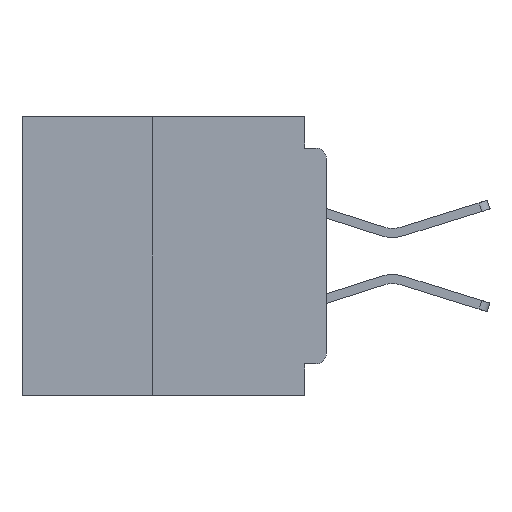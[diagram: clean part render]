
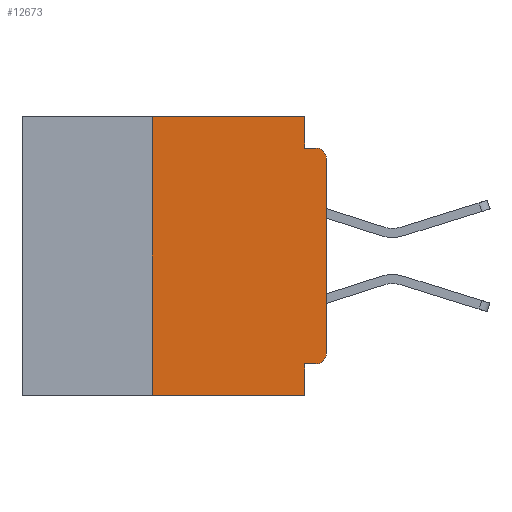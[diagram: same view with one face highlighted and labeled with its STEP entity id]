
A CAD part, left-side view. The second image highlights one B-rep face of the part: STEP entity #12673.
In plain terms, the highlighted planar face has unit normal (-1, 0, 0).
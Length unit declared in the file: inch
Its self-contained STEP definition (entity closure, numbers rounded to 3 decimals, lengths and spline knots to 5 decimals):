
#112 = CARTESIAN_POINT ( 'NONE',  ( 0., 0., -0.355 ) ) ;
#574 = CARTESIAN_POINT ( 'NONE',  ( 0., 0.437, -0.4 ) ) ;
#631 = VERTEX_POINT ( 'NONE', #1686 ) ;
#1043 = EDGE_CURVE ( 'NONE', #2421, #39814, #21181, .T. ) ;
#1280 = VECTOR ( 'NONE', #12761, 39.37008 ) ;
#1314 = CARTESIAN_POINT ( 'NONE',  ( 0., 0.015, -0.045 ) ) ;
#1686 = CARTESIAN_POINT ( 'NONE',  ( 0., 0.031, -0.355 ) ) ;
#2421 = VERTEX_POINT ( 'NONE', #5644 ) ;
#2426 = LINE ( 'NONE', #34821, #18251 ) ;
#3093 = CARTESIAN_POINT ( 'NONE',  ( 0., 0.25, -0.4 ) ) ;
#3097 = CARTESIAN_POINT ( 'NONE',  ( 0., 0.031, -0.4 ) ) ;
#3476 = CARTESIAN_POINT ( 'NONE',  ( 0., 0.015, -0.06 ) ) ;
#3678 = EDGE_CURVE ( 'NONE', #27109, #631, #16593, .T. ) ;
#3680 = CARTESIAN_POINT ( 'NONE',  ( 0., 0.031, 0. ) ) ;
#3747 = PLANE ( 'NONE',  #7463 ) ;
#3803 = DIRECTION ( 'NONE',  ( 0., -1., 0. ) ) ;
#4270 = CARTESIAN_POINT ( 'NONE',  ( 0., 0., -0.06 ) ) ;
#4864 = VERTEX_POINT ( 'NONE', #4270 ) ;
#4935 = CARTESIAN_POINT ( 'NONE',  ( 0., 0.031, 0. ) ) ;
#5644 = CARTESIAN_POINT ( 'NONE',  ( 0., 0.031, -0.045 ) ) ;
#6424 = VECTOR ( 'NONE', #35886, 39.37008 ) ;
#6464 = EDGE_CURVE ( 'NONE', #8385, #29759, #18875, .T. ) ;
#6655 = DIRECTION ( 'NONE',  ( 0., 0., -1. ) ) ;
#6910 = DIRECTION ( 'NONE',  ( 0., 0., -1. ) ) ;
#6950 = CIRCLE ( 'NONE', #19145, 0.015 ) ;
#7463 = AXIS2_PLACEMENT_3D ( 'NONE', #22542, #25592, #6910 ) ;
#7711 = ORIENTED_EDGE ( 'NONE', *, *, #16539, .T. ) ;
#7778 = FACE_OUTER_BOUND ( 'NONE', #20797, .T. ) ;
#8385 = VERTEX_POINT ( 'NONE', #12270 ) ;
#8559 = VECTOR ( 'NONE', #3803, 39.37008 ) ;
#9149 = EDGE_CURVE ( 'NONE', #31643, #25227, #2426, .T. ) ;
#9467 = DIRECTION ( 'NONE',  ( 0., 0., 1. ) ) ;
#9840 = ORIENTED_EDGE ( 'NONE', *, *, #20306, .T. ) ;
#9874 = ORIENTED_EDGE ( 'NONE', *, *, #1043, .F. ) ;
#9948 = CARTESIAN_POINT ( 'NONE',  ( 0., 0.015, -0.34 ) ) ;
#11998 = CARTESIAN_POINT ( 'NONE',  ( 0., 0.031, -0.4 ) ) ;
#12270 = CARTESIAN_POINT ( 'NONE',  ( 0., 0.25, -0.4 ) ) ;
#12673 = ADVANCED_FACE ( 'NONE', ( #7778 ), #3747, .F. ) ;
#12761 = DIRECTION ( 'NONE',  ( 0., 0., -1. ) ) ;
#13107 = DIRECTION ( 'NONE',  ( 0., 0., -1. ) ) ;
#14820 = LINE ( 'NONE', #4935, #6424 ) ;
#15845 = CARTESIAN_POINT ( 'NONE',  ( 0., 0.015, -0.355 ) ) ;
#16113 = LINE ( 'NONE', #3093, #31457 ) ;
#16539 = EDGE_CURVE ( 'NONE', #4864, #39814, #6950, .T. ) ;
#16593 = LINE ( 'NONE', #112, #39059 ) ;
#17129 = LINE ( 'NONE', #3097, #1280 ) ;
#18251 = VECTOR ( 'NONE', #25818, 39.37008 ) ;
#18295 = VECTOR ( 'NONE', #37174, 39.37008 ) ;
#18869 = CARTESIAN_POINT ( 'NONE',  ( 0., 0., 0. ) ) ;
#18875 = LINE ( 'NONE', #574, #8559 ) ;
#19145 = AXIS2_PLACEMENT_3D ( 'NONE', #3476, #25351, #6655 ) ;
#20306 = EDGE_CURVE ( 'NONE', #27109, #23958, #23934, .T. ) ;
#20797 = EDGE_LOOP ( 'NONE', ( #24106, #7711, #9874, #38422, #25139, #29054, #37532, #32248, #30099, #9840 ) ) ;
#21181 = LINE ( 'NONE', #21753, #37399 ) ;
#21360 = EDGE_CURVE ( 'NONE', #8385, #31643, #16113, .T. ) ;
#21753 = CARTESIAN_POINT ( 'NONE',  ( 0., 0., -0.045 ) ) ;
#22542 = CARTESIAN_POINT ( 'NONE',  ( 0., 0.437, 0. ) ) ;
#23934 = CIRCLE ( 'NONE', #32503, 0.015 ) ;
#23958 = VERTEX_POINT ( 'NONE', #37731 ) ;
#24106 = ORIENTED_EDGE ( 'NONE', *, *, #39456, .T. ) ;
#25139 = ORIENTED_EDGE ( 'NONE', *, *, #9149, .F. ) ;
#25227 = VERTEX_POINT ( 'NONE', #3680 ) ;
#25351 = DIRECTION ( 'NONE',  ( -1., 0., 0. ) ) ;
#25592 = DIRECTION ( 'NONE',  ( 1., 0., 0. ) ) ;
#25818 = DIRECTION ( 'NONE',  ( 0., -1., 0. ) ) ;
#27109 = VERTEX_POINT ( 'NONE', #15845 ) ;
#29054 = ORIENTED_EDGE ( 'NONE', *, *, #21360, .F. ) ;
#29759 = VERTEX_POINT ( 'NONE', #11998 ) ;
#30099 = ORIENTED_EDGE ( 'NONE', *, *, #3678, .F. ) ;
#31457 = VECTOR ( 'NONE', #9467, 39.37008 ) ;
#31562 = DIRECTION ( 'NONE',  ( -1., 0., 0. ) ) ;
#31643 = VERTEX_POINT ( 'NONE', #38542 ) ;
#32248 = ORIENTED_EDGE ( 'NONE', *, *, #34902, .F. ) ;
#32503 = AXIS2_PLACEMENT_3D ( 'NONE', #9948, #31562, #13107 ) ;
#32600 = LINE ( 'NONE', #18869, #18295 ) ;
#33229 = DIRECTION ( 'NONE',  ( 0., -1., 0. ) ) ;
#33464 = EDGE_CURVE ( 'NONE', #25227, #2421, #14820, .T. ) ;
#34821 = CARTESIAN_POINT ( 'NONE',  ( 0., 0.437, 0. ) ) ;
#34902 = EDGE_CURVE ( 'NONE', #631, #29759, #17129, .T. ) ;
#35093 = DIRECTION ( 'NONE',  ( 0., 1., 0. ) ) ;
#35886 = DIRECTION ( 'NONE',  ( 0., 0., -1. ) ) ;
#37174 = DIRECTION ( 'NONE',  ( 0., 0., 1. ) ) ;
#37399 = VECTOR ( 'NONE', #33229, 39.37008 ) ;
#37532 = ORIENTED_EDGE ( 'NONE', *, *, #6464, .T. ) ;
#37731 = CARTESIAN_POINT ( 'NONE',  ( 0., 0., -0.34 ) ) ;
#38422 = ORIENTED_EDGE ( 'NONE', *, *, #33464, .F. ) ;
#38542 = CARTESIAN_POINT ( 'NONE',  ( 0., 0.25, 0. ) ) ;
#39059 = VECTOR ( 'NONE', #35093, 39.37008 ) ;
#39456 = EDGE_CURVE ( 'NONE', #23958, #4864, #32600, .T. ) ;
#39814 = VERTEX_POINT ( 'NONE', #1314 ) ;
